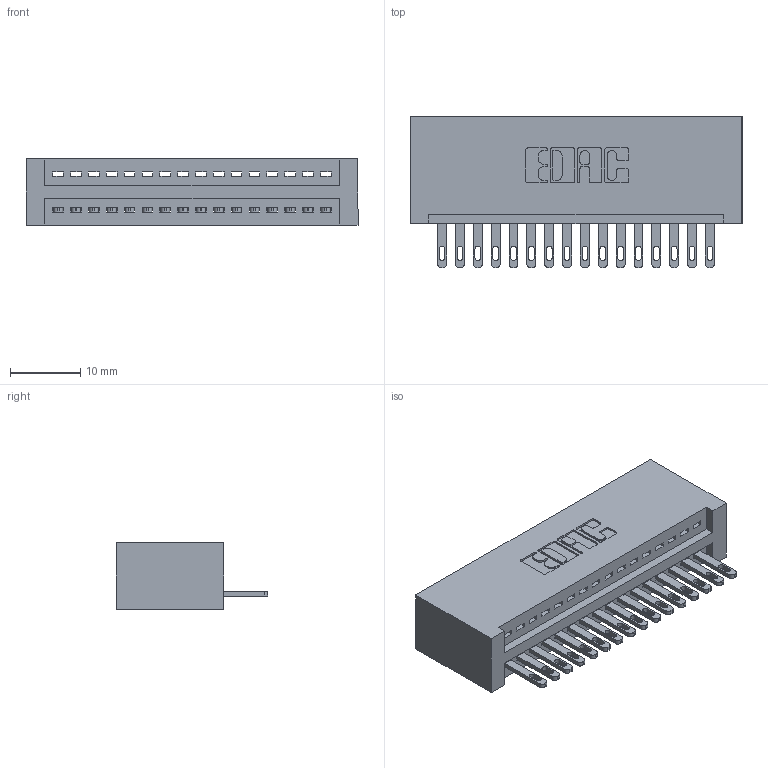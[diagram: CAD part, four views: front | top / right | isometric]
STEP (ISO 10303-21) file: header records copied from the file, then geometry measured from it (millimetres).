
FILE_DESCRIPTION (( 'STEP AP203' ), '1' );
FILE_NAME ('895-016-500-101.STEP', '2020-09-25T04:13:11', ( '' ), ( '' ), 'SwSTEP 2.0', 'SolidWorks 2020', '' );
FILE_SCHEMA (( 'CONFIG_CONTROL_DESIGN' ));
Length unit declared in the file: inch
Products named in the file (3): 845 Part_No Mounting Lugs; 345-292-001_345-293-100; 895-016-500-101
Assembly tree (17 placements, depth 2):
  895-016-500-101
    845 Part_No Mounting Lugs
    345-292-001_345-293-100  x16
Bounding box: 47.24 x 21.51 x 9.4 mm (x, y, z)
Volume: 4868.6 mm3; surface area: 6342.6 mm2
Topology: 17 solids, 17 shells, 982 faces, 3005 edges, 2002 vertices
Faces by surface type: plane 620, cylinder 362
Entity records: 15195 total; most frequent: CARTESIAN_POINT 2640, ORIENTED_EDGE 2590, DIRECTION 2339, EDGE_CURVE 1295, VECTOR 1103, LINE 1103, VERTEX_POINT 862, AXIS2_PLACEMENT_3D 618
